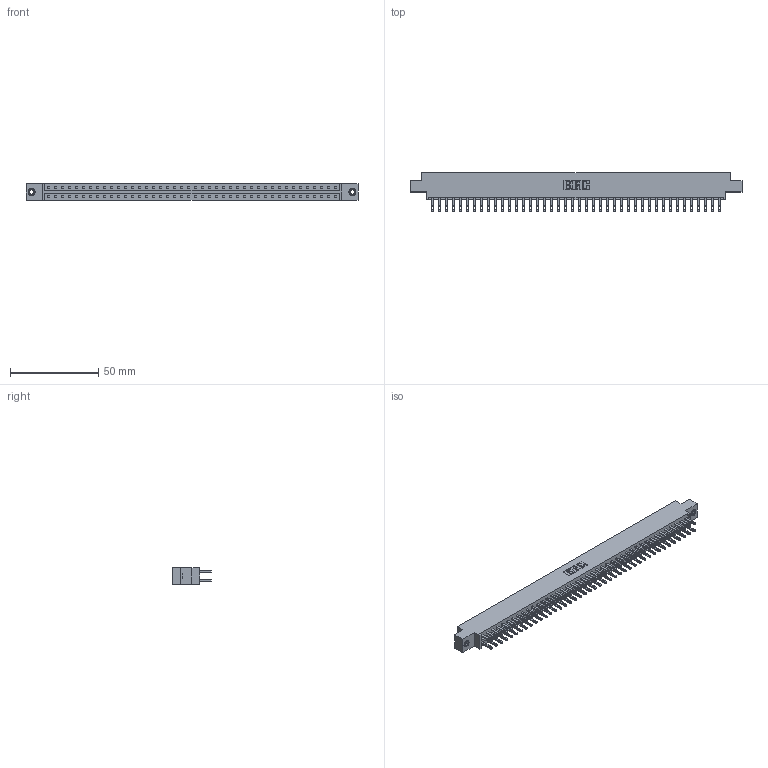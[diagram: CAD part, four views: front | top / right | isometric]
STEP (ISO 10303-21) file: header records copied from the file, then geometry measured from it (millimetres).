
FILE_DESCRIPTION (( 'STEP AP203' ), '1' );
FILE_NAME ('833-084-500-807.STEP', '2020-06-06T00:47:54', ( '' ), ( '' ), 'SwSTEP 2.0', 'SolidWorks 2020', '' );
FILE_SCHEMA (( 'CONFIG_CONTROL_DESIGN' ));
Length unit declared in the file: inch
Products named in the file (4): 345-292-001_345-293-100; 833 Part_Offset - .156 Dia - TI; 833-084-500-807; 345-250-001_345-250-005-103
Assembly tree (87 placements, depth 2):
  833-084-500-807
    833 Part_Offset - .156 Dia - TI
    345-292-001_345-293-100  x84
    345-250-001_345-250-005-103  x2
Bounding box: 187.96 x 21.85 x 9.4 mm (x, y, z)
Volume: 19205 mm3; surface area: 23884.4 mm2
Topology: 87 solids, 87 shells, 4210 faces, 12807 edges, 8530 vertices
Faces by surface type: plane 2626, cylinder 1568, cone 12, torus 4
Entity records: 28268 total; most frequent: CARTESIAN_POINT 4669, ORIENTED_EDGE 4598, DIRECTION 4021, EDGE_CURVE 2299, VECTOR 2147, LINE 2147, VERTEX_POINT 1528, AXIS2_PLACEMENT_3D 937
